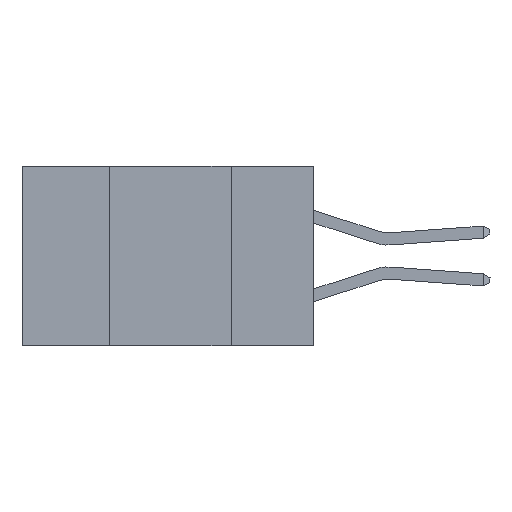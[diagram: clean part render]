
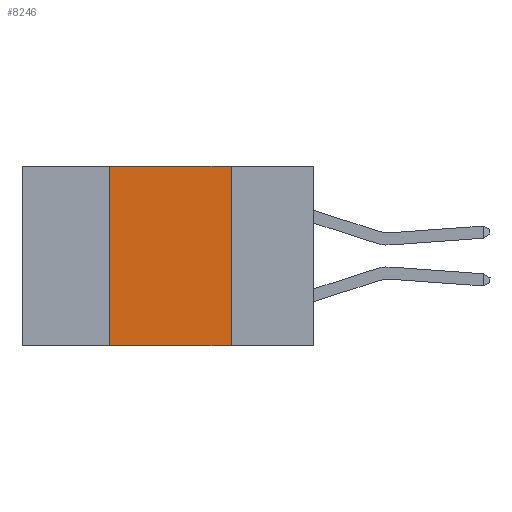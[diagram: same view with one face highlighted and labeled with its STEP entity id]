
A CAD part, left-side view. The second image highlights one B-rep face of the part: STEP entity #8246.
In plain terms, the highlighted planar face has unit normal (-1, 0, 0).
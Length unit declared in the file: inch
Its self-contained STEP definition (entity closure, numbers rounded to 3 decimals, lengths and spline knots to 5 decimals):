
#319 = CARTESIAN_POINT ( 'NONE',  ( 0., 0.6, 0. ) ) ;
#666 = CARTESIAN_POINT ( 'NONE',  ( 0., 0.6, -0.37 ) ) ;
#673 = DIRECTION ( 'NONE',  ( 0., -1., 0. ) ) ;
#961 = DIRECTION ( 'NONE',  ( 0., 0., -1. ) ) ;
#1137 = VERTEX_POINT ( 'NONE', #6249 ) ;
#1177 = ORIENTED_EDGE ( 'NONE', *, *, #6832, .F. ) ;
#1181 = DIRECTION ( 'NONE',  ( 0., -1., 0. ) ) ;
#1551 = AXIS2_PLACEMENT_3D ( 'NONE', #2254, #1912, #4831 ) ;
#1641 = VECTOR ( 'NONE', #961, 39.37008 ) ;
#1912 = DIRECTION ( 'NONE',  ( 1., 0., 0. ) ) ;
#1994 = DIRECTION ( 'NONE',  ( 0., 0., 1. ) ) ;
#2254 = CARTESIAN_POINT ( 'NONE',  ( 0., 0.6, 0. ) ) ;
#2580 = CARTESIAN_POINT ( 'NONE',  ( 0., 0.17, 0. ) ) ;
#2786 = VECTOR ( 'NONE', #1181, 39.37008 ) ;
#3175 = CARTESIAN_POINT ( 'NONE',  ( 0., 0.42, 0. ) ) ;
#3776 = LINE ( 'NONE', #2580, #1641 ) ;
#4591 = VERTEX_POINT ( 'NONE', #8807 ) ;
#4752 = PLANE ( 'NONE',  #1551 ) ;
#4831 = DIRECTION ( 'NONE',  ( 0., 0., -1. ) ) ;
#5644 = EDGE_CURVE ( 'NONE', #4591, #5855, #3776, .T. ) ;
#5855 = VERTEX_POINT ( 'NONE', #5904 ) ;
#5904 = CARTESIAN_POINT ( 'NONE',  ( 0., 0.17, -0.37 ) ) ;
#6067 = LINE ( 'NONE', #3175, #8037 ) ;
#6089 = EDGE_CURVE ( 'NONE', #1137, #6477, #6067, .T. ) ;
#6156 = VECTOR ( 'NONE', #673, 39.37008 ) ;
#6249 = CARTESIAN_POINT ( 'NONE',  ( 0., 0.42, -0.37 ) ) ;
#6383 = LINE ( 'NONE', #319, #6156 ) ;
#6398 = ORIENTED_EDGE ( 'NONE', *, *, #6551, .T. ) ;
#6477 = VERTEX_POINT ( 'NONE', #8280 ) ;
#6551 = EDGE_CURVE ( 'NONE', #1137, #5855, #8247, .T. ) ;
#6603 = ORIENTED_EDGE ( 'NONE', *, *, #6089, .F. ) ;
#6832 = EDGE_CURVE ( 'NONE', #6477, #4591, #6383, .T. ) ;
#7113 = EDGE_LOOP ( 'NONE', ( #7415, #1177, #6603, #6398 ) ) ;
#7415 = ORIENTED_EDGE ( 'NONE', *, *, #5644, .F. ) ;
#7681 = FACE_OUTER_BOUND ( 'NONE', #7113, .T. ) ;
#8037 = VECTOR ( 'NONE', #1994, 39.37008 ) ;
#8246 = ADVANCED_FACE ( 'NONE', ( #7681 ), #4752, .F. ) ;
#8247 = LINE ( 'NONE', #666, #2786 ) ;
#8280 = CARTESIAN_POINT ( 'NONE',  ( 0., 0.42, 0. ) ) ;
#8807 = CARTESIAN_POINT ( 'NONE',  ( 0., 0.17, 0. ) ) ;
